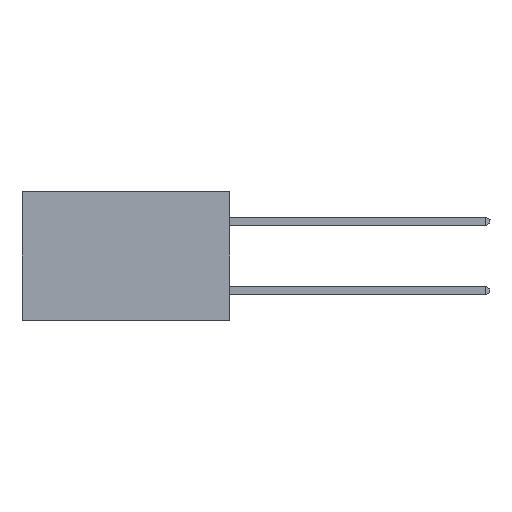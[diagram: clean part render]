
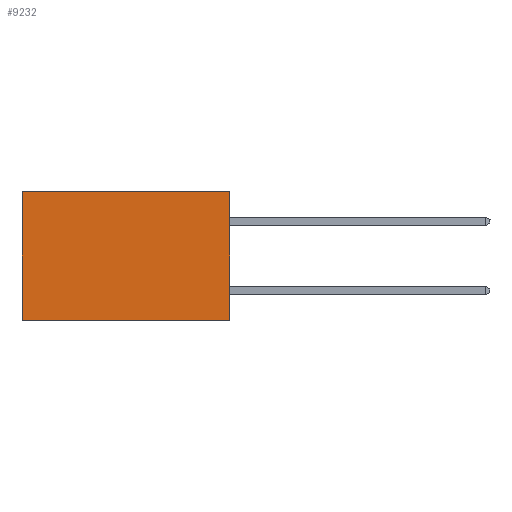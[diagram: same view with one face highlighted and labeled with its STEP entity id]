
A CAD part, left-side view. The second image highlights one B-rep face of the part: STEP entity #9232.
In plain terms, the highlighted planar face has unit normal (-1, 0, 0).
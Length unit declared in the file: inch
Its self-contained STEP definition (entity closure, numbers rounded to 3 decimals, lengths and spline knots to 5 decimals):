
#842 = VERTEX_POINT ( 'NONE', #2835 ) ;
#1335 = ORIENTED_EDGE ( 'NONE', *, *, #6674, .F. ) ;
#1358 = LINE ( 'NONE', #1549, #1592 ) ;
#1549 = CARTESIAN_POINT ( 'NONE',  ( 0.298, 0., 0. ) ) ;
#1592 = VECTOR ( 'NONE', #2412, 39.37008 ) ;
#1616 = AXIS2_PLACEMENT_3D ( 'NONE', #3214, #5517, #6267 ) ;
#2017 = DIRECTION ( 'NONE',  ( 0., 1., 0. ) ) ;
#2412 = DIRECTION ( 'NONE',  ( 0., 0., -1. ) ) ;
#2835 = CARTESIAN_POINT ( 'NONE',  ( 0.298, 0.6, 0. ) ) ;
#3039 = VECTOR ( 'NONE', #3995, 39.37008 ) ;
#3214 = CARTESIAN_POINT ( 'NONE',  ( 0.298, 0., 0. ) ) ;
#3341 = EDGE_LOOP ( 'NONE', ( #4498, #1335, #4835, #5675 ) ) ;
#3995 = DIRECTION ( 'NONE',  ( 0., 1., 0. ) ) ;
#4438 = VERTEX_POINT ( 'NONE', #5375 ) ;
#4498 = ORIENTED_EDGE ( 'NONE', *, *, #9579, .T. ) ;
#4835 = ORIENTED_EDGE ( 'NONE', *, *, #9677, .F. ) ;
#4849 = VERTEX_POINT ( 'NONE', #5820 ) ;
#5256 = CARTESIAN_POINT ( 'NONE',  ( 0.298, 0.6, 0. ) ) ;
#5375 = CARTESIAN_POINT ( 'NONE',  ( 0.298, 0., 0. ) ) ;
#5466 = CARTESIAN_POINT ( 'NONE',  ( 0.298, 0., -0.37 ) ) ;
#5517 = DIRECTION ( 'NONE',  ( 1., 0., 0. ) ) ;
#5570 = VECTOR ( 'NONE', #6705, 39.37008 ) ;
#5675 = ORIENTED_EDGE ( 'NONE', *, *, #6726, .T. ) ;
#5807 = FACE_OUTER_BOUND ( 'NONE', #3341, .T. ) ;
#5820 = CARTESIAN_POINT ( 'NONE',  ( 0.298, 0., -0.37 ) ) ;
#6267 = DIRECTION ( 'NONE',  ( 0., 0., -1. ) ) ;
#6356 = CARTESIAN_POINT ( 'NONE',  ( 0.298, 0.6, -0.37 ) ) ;
#6674 = EDGE_CURVE ( 'NONE', #4849, #9410, #7741, .T. ) ;
#6705 = DIRECTION ( 'NONE',  ( 0., 0., -1. ) ) ;
#6726 = EDGE_CURVE ( 'NONE', #4438, #842, #7050, .T. ) ;
#6766 = LINE ( 'NONE', #5256, #5570 ) ;
#7050 = LINE ( 'NONE', #9469, #8796 ) ;
#7741 = LINE ( 'NONE', #5466, #3039 ) ;
#8796 = VECTOR ( 'NONE', #2017, 39.37008 ) ;
#8984 = PLANE ( 'NONE',  #1616 ) ;
#9232 = ADVANCED_FACE ( 'NONE', ( #5807 ), #8984, .F. ) ;
#9410 = VERTEX_POINT ( 'NONE', #6356 ) ;
#9469 = CARTESIAN_POINT ( 'NONE',  ( 0.298, 0., 0. ) ) ;
#9579 = EDGE_CURVE ( 'NONE', #842, #9410, #6766, .T. ) ;
#9677 = EDGE_CURVE ( 'NONE', #4438, #4849, #1358, .T. ) ;
